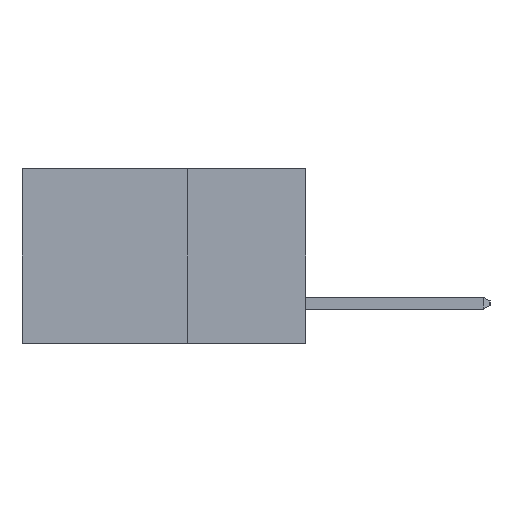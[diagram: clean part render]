
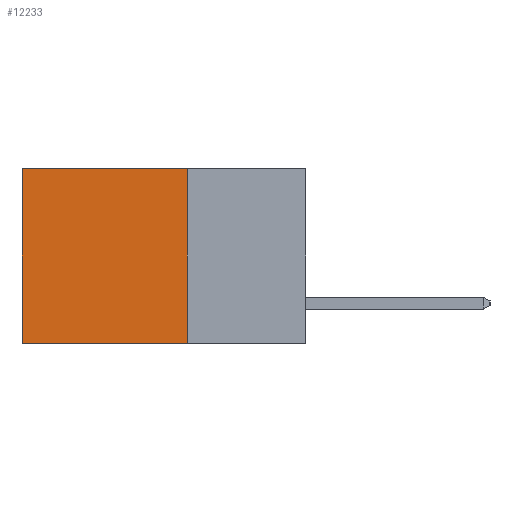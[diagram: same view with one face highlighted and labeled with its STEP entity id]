
A CAD part, left-side view. The second image highlights one B-rep face of the part: STEP entity #12233.
In plain terms, the highlighted planar face has unit normal (-1, 0, 0).
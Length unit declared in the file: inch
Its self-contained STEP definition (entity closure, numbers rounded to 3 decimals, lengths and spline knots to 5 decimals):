
#681 = DIRECTION ( 'NONE',  ( 0., 0., -1. ) ) ;
#806 = EDGE_CURVE ( 'NONE', #1502, #13337, #12467, .T. ) ;
#1000 = CARTESIAN_POINT ( 'NONE',  ( 0.298, 0.25, -0.37 ) ) ;
#1502 = VERTEX_POINT ( 'NONE', #2108 ) ;
#1730 = EDGE_LOOP ( 'NONE', ( #6098, #7569, #1822, #4303 ) ) ;
#1747 = PLANE ( 'NONE',  #5399 ) ;
#1822 = ORIENTED_EDGE ( 'NONE', *, *, #11420, .F. ) ;
#1903 = LINE ( 'NONE', #12977, #10252 ) ;
#2108 = CARTESIAN_POINT ( 'NONE',  ( 0.298, 0.6, 0. ) ) ;
#2151 = VECTOR ( 'NONE', #12360, 39.37008 ) ;
#2411 = VERTEX_POINT ( 'NONE', #3899 ) ;
#3505 = DIRECTION ( 'NONE',  ( 0., 1., 0. ) ) ;
#3899 = CARTESIAN_POINT ( 'NONE',  ( 0.298, 0.25, 0. ) ) ;
#4097 = EDGE_CURVE ( 'NONE', #13735, #13337, #1903, .T. ) ;
#4303 = ORIENTED_EDGE ( 'NONE', *, *, #5507, .T. ) ;
#4313 = LINE ( 'NONE', #13132, #9694 ) ;
#5073 = CARTESIAN_POINT ( 'NONE',  ( 0.298, 0.6, 0. ) ) ;
#5399 = AXIS2_PLACEMENT_3D ( 'NONE', #11518, #7231, #681 ) ;
#5507 = EDGE_CURVE ( 'NONE', #2411, #1502, #4313, .T. ) ;
#5737 = LINE ( 'NONE', #10236, #2151 ) ;
#6098 = ORIENTED_EDGE ( 'NONE', *, *, #806, .T. ) ;
#7231 = DIRECTION ( 'NONE',  ( 1., 0., 0. ) ) ;
#7434 = VECTOR ( 'NONE', #9137, 39.37008 ) ;
#7569 = ORIENTED_EDGE ( 'NONE', *, *, #4097, .F. ) ;
#7637 = DIRECTION ( 'NONE',  ( 0., 1., 0. ) ) ;
#8968 = CARTESIAN_POINT ( 'NONE',  ( 0.298, 0.6, -0.37 ) ) ;
#9137 = DIRECTION ( 'NONE',  ( 0., 0., -1. ) ) ;
#9694 = VECTOR ( 'NONE', #3505, 39.37008 ) ;
#10236 = CARTESIAN_POINT ( 'NONE',  ( 0.298, 0.25, 0. ) ) ;
#10252 = VECTOR ( 'NONE', #7637, 39.37008 ) ;
#11420 = EDGE_CURVE ( 'NONE', #2411, #13735, #5737, .T. ) ;
#11518 = CARTESIAN_POINT ( 'NONE',  ( 0.298, 0.25, 0. ) ) ;
#12233 = ADVANCED_FACE ( 'NONE', ( #13443 ), #1747, .F. ) ;
#12360 = DIRECTION ( 'NONE',  ( 0., 0., -1. ) ) ;
#12467 = LINE ( 'NONE', #5073, #7434 ) ;
#12977 = CARTESIAN_POINT ( 'NONE',  ( 0.298, 0.25, -0.37 ) ) ;
#13132 = CARTESIAN_POINT ( 'NONE',  ( 0.298, 0.25, 0. ) ) ;
#13337 = VERTEX_POINT ( 'NONE', #8968 ) ;
#13443 = FACE_OUTER_BOUND ( 'NONE', #1730, .T. ) ;
#13735 = VERTEX_POINT ( 'NONE', #1000 ) ;
